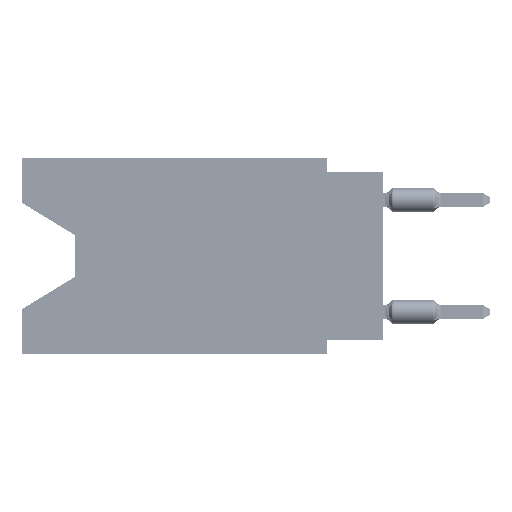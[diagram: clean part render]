
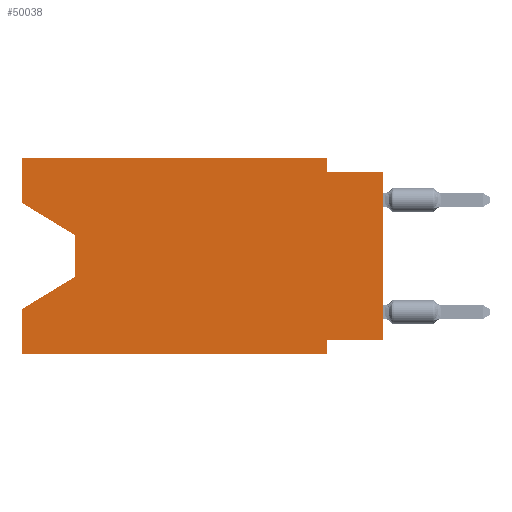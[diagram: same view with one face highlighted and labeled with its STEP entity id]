
A CAD part, left-side view. The second image highlights one B-rep face of the part: STEP entity #50038.
In plain terms, the highlighted planar face has unit normal (-1, 0, 0).
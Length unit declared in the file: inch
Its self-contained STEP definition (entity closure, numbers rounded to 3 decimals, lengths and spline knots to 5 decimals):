
#426 = CARTESIAN_POINT ( 'NONE',  ( 0., 0., 0. ) ) ;
#915 = CARTESIAN_POINT ( 'NONE',  ( 0., 0., -0.025 ) ) ;
#1053 = VECTOR ( 'NONE', #14783, 39.37008 ) ;
#1334 = ORIENTED_EDGE ( 'NONE', *, *, #26840, .T. ) ;
#1379 = CARTESIAN_POINT ( 'NONE',  ( 0., 0.645, -0.26975 ) ) ;
#2630 = VECTOR ( 'NONE', #36227, 39.37008 ) ;
#2797 = DIRECTION ( 'NONE',  ( 0., 0.855, -0.519 ) ) ;
#2887 = ORIENTED_EDGE ( 'NONE', *, *, #61389, .T. ) ;
#4681 = EDGE_LOOP ( 'NONE', ( #1334, #19913, #29860, #25337, #2887, #49406, #48184, #34853, #10886, #27536, #46761, #52339 ) ) ;
#5264 = EDGE_CURVE ( 'NONE', #13056, #65181, #16696, .T. ) ;
#5279 = VERTEX_POINT ( 'NONE', #52190 ) ;
#5932 = DIRECTION ( 'NONE',  ( 1., 0., 0. ) ) ;
#6885 = LINE ( 'NONE', #31279, #7213 ) ;
#6901 = EDGE_CURVE ( 'NONE', #52860, #13280, #35519, .T. ) ;
#7008 = CARTESIAN_POINT ( 'NONE',  ( 0., 0.1, 0. ) ) ;
#7213 = VECTOR ( 'NONE', #41653, 39.37008 ) ;
#7649 = VERTEX_POINT ( 'NONE', #55068 ) ;
#10417 = VERTEX_POINT ( 'NONE', #18910 ) ;
#10886 = ORIENTED_EDGE ( 'NONE', *, *, #57201, .F. ) ;
#11050 = VECTOR ( 'NONE', #20817, 39.37008 ) ;
#11276 = FACE_OUTER_BOUND ( 'NONE', #4681, .T. ) ;
#12261 = DIRECTION ( 'NONE',  ( 0., 0., 1. ) ) ;
#12928 = LINE ( 'NONE', #13270, #53893 ) ;
#13056 = VERTEX_POINT ( 'NONE', #35839 ) ;
#13270 = CARTESIAN_POINT ( 'NONE',  ( 0., 0.645, 0. ) ) ;
#13280 = VERTEX_POINT ( 'NONE', #915 ) ;
#14783 = DIRECTION ( 'NONE',  ( 0., 0., 1. ) ) ;
#15849 = LINE ( 'NONE', #40908, #2630 ) ;
#16122 = VECTOR ( 'NONE', #2797, 39.37008 ) ;
#16696 = LINE ( 'NONE', #7008, #47675 ) ;
#16851 = VERTEX_POINT ( 'NONE', #60578 ) ;
#17374 = VERTEX_POINT ( 'NONE', #61814 ) ;
#18065 = EDGE_CURVE ( 'NONE', #5279, #10417, #36953, .T. ) ;
#18910 = CARTESIAN_POINT ( 'NONE',  ( 0., 0.55, -0.212 ) ) ;
#19913 = ORIENTED_EDGE ( 'NONE', *, *, #18065, .T. ) ;
#20817 = DIRECTION ( 'NONE',  ( 0., 0., 1. ) ) ;
#23893 = DIRECTION ( 'NONE',  ( 0., -1., 0. ) ) ;
#24089 = EDGE_CURVE ( 'NONE', #35499, #17374, #30777, .T. ) ;
#24412 = DIRECTION ( 'NONE',  ( 0., -1., 0. ) ) ;
#25265 = LINE ( 'NONE', #47670, #49049 ) ;
#25337 = ORIENTED_EDGE ( 'NONE', *, *, #62673, .F. ) ;
#26581 = CARTESIAN_POINT ( 'NONE',  ( 0., 0.55, -0.138 ) ) ;
#26840 = EDGE_CURVE ( 'NONE', #16851, #5279, #15849, .T. ) ;
#27536 = ORIENTED_EDGE ( 'NONE', *, *, #5264, .F. ) ;
#29422 = LINE ( 'NONE', #50859, #44419 ) ;
#29467 = DIRECTION ( 'NONE',  ( 0., 0., -1. ) ) ;
#29860 = ORIENTED_EDGE ( 'NONE', *, *, #34323, .T. ) ;
#30777 = LINE ( 'NONE', #35457, #63346 ) ;
#31279 = CARTESIAN_POINT ( 'NONE',  ( 0., 0., -0.025 ) ) ;
#31312 = PLANE ( 'NONE',  #39918 ) ;
#31589 = DIRECTION ( 'NONE',  ( 0., 1., 0. ) ) ;
#33046 = VERTEX_POINT ( 'NONE', #1379 ) ;
#34323 = EDGE_CURVE ( 'NONE', #10417, #33046, #61698, .T. ) ;
#34853 = ORIENTED_EDGE ( 'NONE', *, *, #6901, .T. ) ;
#35457 = CARTESIAN_POINT ( 'NONE',  ( 0., 0.1, -0.35 ) ) ;
#35499 = VERTEX_POINT ( 'NONE', #54695 ) ;
#35519 = LINE ( 'NONE', #426, #11050 ) ;
#35839 = CARTESIAN_POINT ( 'NONE',  ( 0., 0.1, 0. ) ) ;
#36227 = DIRECTION ( 'NONE',  ( 0., -0.855, -0.519 ) ) ;
#36953 = LINE ( 'NONE', #26581, #37761 ) ;
#37761 = VECTOR ( 'NONE', #47014, 39.37008 ) ;
#39918 = AXIS2_PLACEMENT_3D ( 'NONE', #51764, #5932, #61463 ) ;
#40908 = CARTESIAN_POINT ( 'NONE',  ( 0., 0.645, -0.08025 ) ) ;
#41453 = DIRECTION ( 'NONE',  ( 0., 0., -1. ) ) ;
#41653 = DIRECTION ( 'NONE',  ( 0., -1., 0. ) ) ;
#43050 = EDGE_CURVE ( 'NONE', #52860, #35499, #25265, .T. ) ;
#43924 = CARTESIAN_POINT ( 'NONE',  ( 0., 0., -0.325 ) ) ;
#44419 = VECTOR ( 'NONE', #24412, 39.37008 ) ;
#45481 = CARTESIAN_POINT ( 'NONE',  ( 0., 0.1, -0.025 ) ) ;
#46761 = ORIENTED_EDGE ( 'NONE', *, *, #64273, .F. ) ;
#47014 = DIRECTION ( 'NONE',  ( 0., 0., -1. ) ) ;
#47670 = CARTESIAN_POINT ( 'NONE',  ( 0., 0., -0.325 ) ) ;
#47675 = VECTOR ( 'NONE', #41453, 39.37008 ) ;
#47973 = CARTESIAN_POINT ( 'NONE',  ( 0., 0.55, -0.212 ) ) ;
#48184 = ORIENTED_EDGE ( 'NONE', *, *, #43050, .F. ) ;
#49049 = VECTOR ( 'NONE', #31589, 39.37008 ) ;
#49406 = ORIENTED_EDGE ( 'NONE', *, *, #24089, .F. ) ;
#50026 = LINE ( 'NONE', #55366, #63982 ) ;
#50038 = ADVANCED_FACE ( 'NONE', ( #11276 ), #31312, .F. ) ;
#50231 = EDGE_CURVE ( 'NONE', #16851, #7649, #12928, .T. ) ;
#50859 = CARTESIAN_POINT ( 'NONE',  ( 0., 0.645, 0. ) ) ;
#51764 = CARTESIAN_POINT ( 'NONE',  ( 0., 0.645, 0. ) ) ;
#52190 = CARTESIAN_POINT ( 'NONE',  ( 0., 0.55, -0.138 ) ) ;
#52339 = ORIENTED_EDGE ( 'NONE', *, *, #50231, .F. ) ;
#52860 = VERTEX_POINT ( 'NONE', #43924 ) ;
#53893 = VECTOR ( 'NONE', #12261, 39.37008 ) ;
#54695 = CARTESIAN_POINT ( 'NONE',  ( 0., 0.1, -0.325 ) ) ;
#55068 = CARTESIAN_POINT ( 'NONE',  ( 0., 0.645, 0. ) ) ;
#55366 = CARTESIAN_POINT ( 'NONE',  ( 0., 0.645, -0.35 ) ) ;
#57201 = EDGE_CURVE ( 'NONE', #65181, #13280, #6885, .T. ) ;
#58304 = CARTESIAN_POINT ( 'NONE',  ( 0., 0.645, -0.35 ) ) ;
#60578 = CARTESIAN_POINT ( 'NONE',  ( 0., 0.645, -0.08025 ) ) ;
#60609 = LINE ( 'NONE', #65624, #1053 ) ;
#61389 = EDGE_CURVE ( 'NONE', #64448, #17374, #50026, .T. ) ;
#61463 = DIRECTION ( 'NONE',  ( 0., 0., -1. ) ) ;
#61698 = LINE ( 'NONE', #47973, #16122 ) ;
#61814 = CARTESIAN_POINT ( 'NONE',  ( 0., 0.1, -0.35 ) ) ;
#62673 = EDGE_CURVE ( 'NONE', #64448, #33046, #60609, .T. ) ;
#63346 = VECTOR ( 'NONE', #29467, 39.37008 ) ;
#63982 = VECTOR ( 'NONE', #23893, 39.37008 ) ;
#64273 = EDGE_CURVE ( 'NONE', #7649, #13056, #29422, .T. ) ;
#64448 = VERTEX_POINT ( 'NONE', #58304 ) ;
#65181 = VERTEX_POINT ( 'NONE', #45481 ) ;
#65624 = CARTESIAN_POINT ( 'NONE',  ( 0., 0.645, 0. ) ) ;
